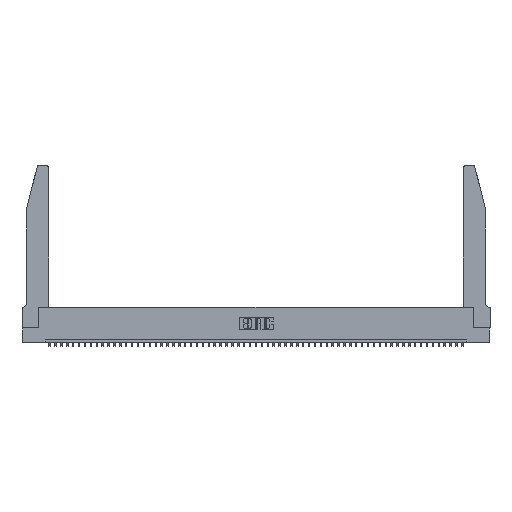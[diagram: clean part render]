
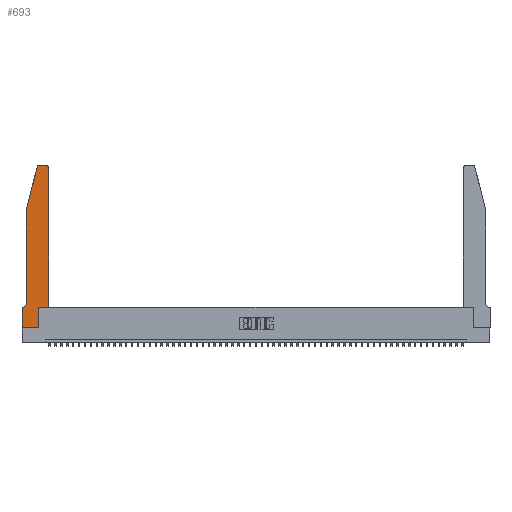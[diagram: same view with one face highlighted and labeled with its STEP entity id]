
A CAD part, top view. The second image highlights one B-rep face of the part: STEP entity #693.
In plain terms, the highlighted planar face has unit normal (0, 0, 1).
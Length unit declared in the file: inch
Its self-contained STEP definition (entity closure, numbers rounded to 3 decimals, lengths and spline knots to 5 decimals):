
#693 = ADVANCED_FACE ( 'NONE', ( #16324 ), #36330, .T. ) ;
#1322 = CARTESIAN_POINT ( 'NONE',  ( 0.0755, 2., 0.37 ) ) ;
#1345 = DIRECTION ( 'NONE',  ( 0., 0., 1. ) ) ;
#1590 = AXIS2_PLACEMENT_3D ( 'NONE', #52476, #43637, #18697 ) ;
#1738 = DIRECTION ( 'NONE',  ( -1., 0., 0. ) ) ;
#1813 = CARTESIAN_POINT ( 'NONE',  ( 0.2605, 2.75, 0.37 ) ) ;
#2399 = VERTEX_POINT ( 'NONE', #26583 ) ;
#2730 = DIRECTION ( 'NONE',  ( -0.239, -0.971, 0. ) ) ;
#3002 = CARTESIAN_POINT ( 'NONE',  ( 0.4505, 2.72, 0.37 ) ) ;
#3007 = ORIENTED_EDGE ( 'NONE', *, *, #22585, .T. ) ;
#3416 = VECTOR ( 'NONE', #41804, 39.37008 ) ;
#3664 = EDGE_CURVE ( 'NONE', #23073, #13504, #37751, .T. ) ;
#4408 = CARTESIAN_POINT ( 'NONE',  ( 0.25487, 2.72718, 0.37 ) ) ;
#4696 = CARTESIAN_POINT ( 'NONE',  ( 0.4505, 0.35, 0.37 ) ) ;
#5041 = CARTESIAN_POINT ( 'NONE',  ( 0.284, 2.75, 0.37 ) ) ;
#5743 = CIRCLE ( 'NONE', #42042, 0.03 ) ;
#5892 = VERTEX_POINT ( 'NONE', #19056 ) ;
#6122 = DIRECTION ( 'NONE',  ( -1., 0., 0. ) ) ;
#6278 = LINE ( 'NONE', #24492, #25966 ) ;
#6602 = CARTESIAN_POINT ( 'NONE',  ( 0., 0.35, 0.37 ) ) ;
#7033 = ORIENTED_EDGE ( 'NONE', *, *, #28307, .T. ) ;
#8231 = VECTOR ( 'NONE', #2730, 39.37008 ) ;
#9021 = DIRECTION ( 'NONE',  ( 0., 1., 0. ) ) ;
#9092 = CARTESIAN_POINT ( 'NONE',  ( 0.0755, 0.35, 0.37 ) ) ;
#9549 = EDGE_CURVE ( 'NONE', #40375, #11473, #42848, .T. ) ;
#10112 = VECTOR ( 'NONE', #9021, 39.37008 ) ;
#11131 = EDGE_CURVE ( 'NONE', #2399, #14827, #51806, .T. ) ;
#11473 = VERTEX_POINT ( 'NONE', #22245 ) ;
#12133 = LINE ( 'NONE', #27777, #46791 ) ;
#12673 = CARTESIAN_POINT ( 'NONE',  ( 0., 0., 0.37 ) ) ;
#12741 = CARTESIAN_POINT ( 'NONE',  ( 0.4505, 0.35, 0.37 ) ) ;
#13164 = VERTEX_POINT ( 'NONE', #51611 ) ;
#13504 = VERTEX_POINT ( 'NONE', #1322 ) ;
#14665 = CARTESIAN_POINT ( 'NONE',  ( 0.0055, 0.42, 0.37 ) ) ;
#14710 = LINE ( 'NONE', #12741, #10112 ) ;
#14827 = VERTEX_POINT ( 'NONE', #5041 ) ;
#15629 = CARTESIAN_POINT ( 'NONE',  ( 0.0755, 2., 0.37 ) ) ;
#16324 = FACE_OUTER_BOUND ( 'NONE', #34679, .T. ) ;
#16800 = VERTEX_POINT ( 'NONE', #3002 ) ;
#17161 = CARTESIAN_POINT ( 'NONE',  ( 0., 0., 0.37 ) ) ;
#17291 = EDGE_CURVE ( 'NONE', #11473, #54147, #6278, .T. ) ;
#17435 = VERTEX_POINT ( 'NONE', #4696 ) ;
#18448 = EDGE_CURVE ( 'NONE', #13504, #39166, #12133, .T. ) ;
#18697 = DIRECTION ( 'NONE',  ( 1., 0., 0. ) ) ;
#19056 = CARTESIAN_POINT ( 'NONE',  ( 0.2865, 0., 0.37 ) ) ;
#19709 = EDGE_CURVE ( 'NONE', #54147, #5892, #19912, .T. ) ;
#19912 = LINE ( 'NONE', #17161, #3416 ) ;
#20947 = CARTESIAN_POINT ( 'NONE',  ( 0.2865, 0.35, 0.37 ) ) ;
#21137 = ORIENTED_EDGE ( 'NONE', *, *, #11131, .T. ) ;
#21600 = DIRECTION ( 'NONE',  ( -1., 0., 0. ) ) ;
#22245 = CARTESIAN_POINT ( 'NONE',  ( 0., 0.35, 0.37 ) ) ;
#22585 = EDGE_CURVE ( 'NONE', #13164, #17435, #37307, .T. ) ;
#22851 = CIRCLE ( 'NONE', #1590, 0.03 ) ;
#23073 = VERTEX_POINT ( 'NONE', #4408 ) ;
#23482 = CARTESIAN_POINT ( 'NONE',  ( 0.0755, 0.42, 0.37 ) ) ;
#23879 = ORIENTED_EDGE ( 'NONE', *, *, #33800, .T. ) ;
#24150 = VECTOR ( 'NONE', #39067, 39.37008 ) ;
#24492 = CARTESIAN_POINT ( 'NONE',  ( 0., 0., 0.37 ) ) ;
#24775 = ORIENTED_EDGE ( 'NONE', *, *, #19709, .T. ) ;
#25448 = AXIS2_PLACEMENT_3D ( 'NONE', #6602, #40576, #36535 ) ;
#25966 = VECTOR ( 'NONE', #26055, 39.37008 ) ;
#26055 = DIRECTION ( 'NONE',  ( 0., -1., 0. ) ) ;
#26583 = CARTESIAN_POINT ( 'NONE',  ( 0.4205, 2.75, 0.37 ) ) ;
#26950 = DIRECTION ( 'NONE',  ( 0., 0., -1. ) ) ;
#26983 = DIRECTION ( 'NONE',  ( 0., -1., 0. ) ) ;
#27777 = CARTESIAN_POINT ( 'NONE',  ( 0.0755, 2., 0.37 ) ) ;
#28227 = EDGE_CURVE ( 'NONE', #16800, #2399, #22851, .T. ) ;
#28307 = EDGE_CURVE ( 'NONE', #39166, #40375, #32855, .T. ) ;
#29867 = AXIS2_PLACEMENT_3D ( 'NONE', #14665, #26950, #1738 ) ;
#30407 = ORIENTED_EDGE ( 'NONE', *, *, #3664, .T. ) ;
#32855 = CIRCLE ( 'NONE', #29867, 0.07 ) ;
#33479 = ORIENTED_EDGE ( 'NONE', *, *, #39520, .T. ) ;
#33800 = EDGE_CURVE ( 'NONE', #14827, #23073, #5743, .T. ) ;
#34316 = VECTOR ( 'NONE', #21600, 39.37008 ) ;
#34382 = CARTESIAN_POINT ( 'NONE',  ( 0.0055, 0.35, 0.37 ) ) ;
#34470 = ORIENTED_EDGE ( 'NONE', *, *, #17291, .T. ) ;
#34679 = EDGE_LOOP ( 'NONE', ( #21137, #23879, #30407, #35595, #7033, #46910, #34470, #24775, #33479, #3007, #46300, #42451 ) ) ;
#35028 = DIRECTION ( 'NONE',  ( 1., 0., 0. ) ) ;
#35595 = ORIENTED_EDGE ( 'NONE', *, *, #18448, .T. ) ;
#35599 = VECTOR ( 'NONE', #51107, 39.37008 ) ;
#36330 = PLANE ( 'NONE',  #25448 ) ;
#36535 = DIRECTION ( 'NONE',  ( 1., 0., 0. ) ) ;
#37307 = LINE ( 'NONE', #47132, #24150 ) ;
#37751 = LINE ( 'NONE', #15629, #8231 ) ;
#39067 = DIRECTION ( 'NONE',  ( 1., 0., 0. ) ) ;
#39166 = VERTEX_POINT ( 'NONE', #23482 ) ;
#39520 = EDGE_CURVE ( 'NONE', #5892, #13164, #46750, .T. ) ;
#40375 = VERTEX_POINT ( 'NONE', #34382 ) ;
#40576 = DIRECTION ( 'NONE',  ( 0., 0., 1. ) ) ;
#41804 = DIRECTION ( 'NONE',  ( 1., 0., 0. ) ) ;
#42042 = AXIS2_PLACEMENT_3D ( 'NONE', #51694, #1345, #35028 ) ;
#42451 = ORIENTED_EDGE ( 'NONE', *, *, #28227, .T. ) ;
#42848 = LINE ( 'NONE', #9092, #34316 ) ;
#43637 = DIRECTION ( 'NONE',  ( 0., 0., 1. ) ) ;
#45362 = VECTOR ( 'NONE', #6122, 39.37008 ) ;
#46300 = ORIENTED_EDGE ( 'NONE', *, *, #47038, .T. ) ;
#46750 = LINE ( 'NONE', #20947, #35599 ) ;
#46791 = VECTOR ( 'NONE', #26983, 39.37008 ) ;
#46910 = ORIENTED_EDGE ( 'NONE', *, *, #9549, .T. ) ;
#47038 = EDGE_CURVE ( 'NONE', #17435, #16800, #14710, .T. ) ;
#47132 = CARTESIAN_POINT ( 'NONE',  ( 0.4505, 0.35, 0.37 ) ) ;
#51107 = DIRECTION ( 'NONE',  ( 0., 1., 0. ) ) ;
#51611 = CARTESIAN_POINT ( 'NONE',  ( 0.2865, 0.35, 0.37 ) ) ;
#51694 = CARTESIAN_POINT ( 'NONE',  ( 0.284, 2.72, 0.37 ) ) ;
#51806 = LINE ( 'NONE', #1813, #45362 ) ;
#52476 = CARTESIAN_POINT ( 'NONE',  ( 0.4205, 2.72, 0.37 ) ) ;
#54147 = VERTEX_POINT ( 'NONE', #12673 ) ;
